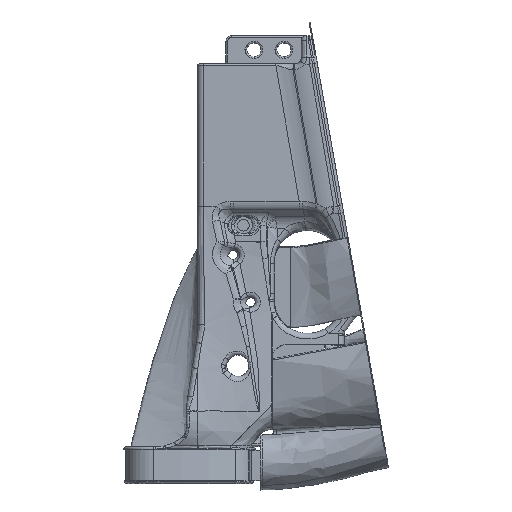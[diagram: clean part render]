
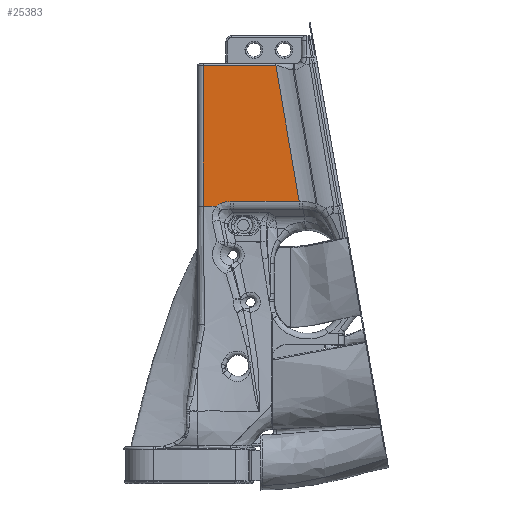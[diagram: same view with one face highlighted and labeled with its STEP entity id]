
A CAD part, left-side view. The second image highlights one B-rep face of the part: STEP entity #25383.
In plain terms, the highlighted planar face has unit normal (-1, 0, 0).
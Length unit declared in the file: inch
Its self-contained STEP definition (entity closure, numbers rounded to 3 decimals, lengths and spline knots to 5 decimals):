
#3293 = CARTESIAN_POINT ( 'NONE',  ( -0.7, -0.49778, 3.70724 ) ) ;
#3439 = DIRECTION ( 'NONE',  ( -1., 0., 0. ) ) ;
#5654 = LINE ( 'NONE', #85281, #105441 ) ;
#6714 = EDGE_CURVE ( 'NONE', #106135, #54826, #5654, .T. ) ;
#6807 = CARTESIAN_POINT ( 'NONE',  ( -0.7, -0.33214, 3.63 ) ) ;
#7147 = ORIENTED_EDGE ( 'NONE', *, *, #109874, .F. ) ;
#8077 = ORIENTED_EDGE ( 'NONE', *, *, #34467, .T. ) ;
#9101 = CARTESIAN_POINT ( 'NONE',  ( -0.7, -0.1, 6.12 ) ) ;
#9178 = CARTESIAN_POINT ( 'NONE',  ( -0.7, -0.33214, 3.63 ) ) ;
#11363 = CARTESIAN_POINT ( 'NONE',  ( -0.7, -0.33214, 3.63 ) ) ;
#12367 = B_SPLINE_CURVE_WITH_KNOTS ( 'NONE', 3,
 ( #6807, #105214, #46326, #30060, #42809, #70200, #98690, #19080, #48237, #116890, #3293, #48874, #118169, #39788 ),
 .UNSPECIFIED., .F., .F.,
 ( 4, 2, 2, 2, 2, 2, 4 ),
 ( 0., 0.00084, 0.00167, 0.00335, 0.00418, 0.00502, 0.00669 ),
 .UNSPECIFIED. ) ;
#17986 = CARTESIAN_POINT ( 'NONE',  ( -0.7, -1.3849, 6.12 ) ) ;
#19080 = CARTESIAN_POINT ( 'NONE',  ( -0.7, -0.45507, 3.69804 ) ) ;
#23135 = B_SPLINE_CURVE_WITH_KNOTS ( 'NONE', 3,
 ( #91498, #44683, #45315, #61713 ),
 .UNSPECIFIED., .F., .F.,
 ( 4, 4 ),
 ( 0.63997, 0.84376 ),
 .UNSPECIFIED. ) ;
#24559 = CARTESIAN_POINT ( 'NONE',  ( -0.7, -0.23042, 3.63 ) ) ;
#25383 = ADVANCED_FACE ( 'NONE', ( #63653 ), #120067, .T. ) ;
#26466 = ORIENTED_EDGE ( 'NONE', *, *, #115775, .F. ) ;
#27163 = B_SPLINE_CURVE_WITH_KNOTS ( 'NONE', 3,
 ( #89610, #98033, #99944, #88963 ),
 .UNSPECIFIED., .F., .F.,
 ( 4, 4 ),
 ( 0.50619, 0.63997 ),
 .UNSPECIFIED. ) ;
#29170 = ORIENTED_EDGE ( 'NONE', *, *, #101780, .T. ) ;
#30060 = CARTESIAN_POINT ( 'NONE',  ( -0.7, -0.366, 3.65781 ) ) ;
#30238 = VERTEX_POINT ( 'NONE', #126111 ) ;
#32839 = LINE ( 'NONE', #111861, #90588 ) ;
#33218 = CARTESIAN_POINT ( 'NONE',  ( -0.7, -2.88773, 6.15 ) ) ;
#34467 = EDGE_CURVE ( 'NONE', #127770, #110384, #118676, .T. ) ;
#36334 = AXIS2_PLACEMENT_3D ( 'NONE', #33218, #3439, #53949 ) ;
#39788 = CARTESIAN_POINT ( 'NONE',  ( -0.7, -0.57376, 3.71284 ) ) ;
#42809 = CARTESIAN_POINT ( 'NONE',  ( -0.7, -0.37527, 3.6638 ) ) ;
#44140 = CARTESIAN_POINT ( 'NONE',  ( -0.7, -0.1, 6.12 ) ) ;
#44683 = CARTESIAN_POINT ( 'NONE',  ( -0.7, -0.18694, 3.63 ) ) ;
#45315 = CARTESIAN_POINT ( 'NONE',  ( -0.70001, -0.14347, 3.63 ) ) ;
#46326 = CARTESIAN_POINT ( 'NONE',  ( -0.7, -0.34834, 3.64474 ) ) ;
#48237 = CARTESIAN_POINT ( 'NONE',  ( -0.7, -0.46573, 3.70081 ) ) ;
#48622 = CARTESIAN_POINT ( 'NONE',  ( -0.7, -0.1, 5.29 ) ) ;
#48874 = CARTESIAN_POINT ( 'NONE',  ( -0.7, -0.5301, 3.71156 ) ) ;
#53713 = CARTESIAN_POINT ( 'NONE',  ( -0.7, -0.1, 4.46 ) ) ;
#53949 = DIRECTION ( 'NONE',  ( 0., 0., 1. ) ) ;
#54826 = VERTEX_POINT ( 'NONE', #44140 ) ;
#60559 = CARTESIAN_POINT ( 'NONE',  ( -0.7, -0.1, 3.63 ) ) ;
#61380 = B_SPLINE_CURVE_WITH_KNOTS ( 'NONE', 3,
 ( #9101, #48622, #53713, #102229 ),
 .UNSPECIFIED., .F., .F.,
 ( 4, 4 ),
 ( -0.15253, -0.08928 ),
 .UNSPECIFIED. ) ;
#61713 = CARTESIAN_POINT ( 'NONE',  ( -0.7, -0.1, 3.63 ) ) ;
#63653 = FACE_OUTER_BOUND ( 'NONE', #105598, .T. ) ;
#64646 = ORIENTED_EDGE ( 'NONE', *, *, #79354, .T. ) ;
#65033 = CARTESIAN_POINT ( 'NONE',  ( -0.7, -1.79804, 3.71284 ) ) ;
#68033 = CARTESIAN_POINT ( 'NONE',  ( -0.7, -0.31604, 3.63 ) ) ;
#68388 = CARTESIAN_POINT ( 'NONE',  ( -0.7, -0.3267, 3.63 ) ) ;
#70200 = CARTESIAN_POINT ( 'NONE',  ( -0.7, -0.40373, 3.67987 ) ) ;
#71553 = DIRECTION ( 'NONE',  ( 0., -1., 0. ) ) ;
#74710 = VERTEX_POINT ( 'NONE', #65033 ) ;
#74915 = DIRECTION ( 'NONE',  ( 0., -1., 0. ) ) ;
#74947 = DIRECTION ( 'NONE',  ( 0., 1., 0. ) ) ;
#76528 = CARTESIAN_POINT ( 'NONE',  ( -0.7, -0.57376, 3.71284 ) ) ;
#76628 = CARTESIAN_POINT ( 'NONE',  ( -0.7, -1.4229, 5.89859 ) ) ;
#79354 = EDGE_CURVE ( 'NONE', #110384, #116969, #12367, .T. ) ;
#85281 = CARTESIAN_POINT ( 'NONE',  ( -0.7, 0., 6.12 ) ) ;
#88498 = ORIENTED_EDGE ( 'NONE', *, *, #6714, .T. ) ;
#88963 = CARTESIAN_POINT ( 'NONE',  ( -0.7, -0.23042, 3.63 ) ) ;
#89610 = CARTESIAN_POINT ( 'NONE',  ( -0.7, -0.31604, 3.63 ) ) ;
#89731 = LINE ( 'NONE', #111068, #122568 ) ;
#90588 = VECTOR ( 'NONE', #74915, 39.37008 ) ;
#91498 = CARTESIAN_POINT ( 'NONE',  ( -0.7, -0.23042, 3.63 ) ) ;
#92084 = ORIENTED_EDGE ( 'NONE', *, *, #108250, .T. ) ;
#97784 = VERTEX_POINT ( 'NONE', #60559 ) ;
#98033 = CARTESIAN_POINT ( 'NONE',  ( -0.69999, -0.2875, 3.63 ) ) ;
#98690 = CARTESIAN_POINT ( 'NONE',  ( -0.7, -0.42375, 3.68828 ) ) ;
#99944 = CARTESIAN_POINT ( 'NONE',  ( -0.7, -0.25896, 3.63 ) ) ;
#101379 = ORIENTED_EDGE ( 'NONE', *, *, #124125, .T. ) ;
#101780 = EDGE_CURVE ( 'NONE', #54826, #97784, #61380, .T. ) ;
#102077 = EDGE_CURVE ( 'NONE', #116969, #30238, #89731, .T. ) ;
#102229 = CARTESIAN_POINT ( 'NONE',  ( -0.7, -0.1, 3.63 ) ) ;
#102526 = ORIENTED_EDGE ( 'NONE', *, *, #102077, .T. ) ;
#105214 = CARTESIAN_POINT ( 'NONE',  ( -0.7, -0.33996, 3.63766 ) ) ;
#105441 = VECTOR ( 'NONE', #74947, 39.37008 ) ;
#105598 = EDGE_LOOP ( 'NONE', ( #8077, #64646, #102526, #92084, #101379, #88498, #29170, #7147, #26466 ) ) ;
#106135 = VERTEX_POINT ( 'NONE', #17986 ) ;
#107035 = LINE ( 'NONE', #76628, #122020 ) ;
#108250 = EDGE_CURVE ( 'NONE', #30238, #74710, #32839, .T. ) ;
#109874 = EDGE_CURVE ( 'NONE', #127936, #97784, #23135, .T. ) ;
#110384 = VERTEX_POINT ( 'NONE', #9178 ) ;
#111068 = CARTESIAN_POINT ( 'NONE',  ( -0.7, -2.88773, 3.71284 ) ) ;
#111861 = CARTESIAN_POINT ( 'NONE',  ( -0.7, -2.88773, 3.71284 ) ) ;
#115775 = EDGE_CURVE ( 'NONE', #127770, #127936, #27163, .T. ) ;
#116890 = CARTESIAN_POINT ( 'NONE',  ( -0.7, -0.48706, 3.7054 ) ) ;
#116969 = VERTEX_POINT ( 'NONE', #76528 ) ;
#117628 = CARTESIAN_POINT ( 'NONE',  ( -0.7, -0.31604, 3.63 ) ) ;
#118169 = CARTESIAN_POINT ( 'NONE',  ( -0.7, -0.55185, 3.71284 ) ) ;
#118676 = B_SPLINE_CURVE_WITH_KNOTS ( 'NONE', 3,
 ( #117628, #118918, #68388, #11363 ),
 .UNSPECIFIED., .F., .F.,
 ( 4, 4 ),
 ( 0., 0.08548 ),
 .UNSPECIFIED. ) ;
#118918 = CARTESIAN_POINT ( 'NONE',  ( -0.7, -0.32137, 3.63 ) ) ;
#120067 = PLANE ( 'NONE',  #36334 ) ;
#122020 = VECTOR ( 'NONE', #127797, 39.37008 ) ;
#122568 = VECTOR ( 'NONE', #71553, 39.37008 ) ;
#124125 = EDGE_CURVE ( 'NONE', #74710, #106135, #107035, .T. ) ;
#126111 = CARTESIAN_POINT ( 'NONE',  ( -0.7, -0.64, 3.71284 ) ) ;
#127770 = VERTEX_POINT ( 'NONE', #68033 ) ;
#127797 = DIRECTION ( 'NONE',  ( 0., 0.169, 0.986 ) ) ;
#127936 = VERTEX_POINT ( 'NONE', #24559 ) ;
